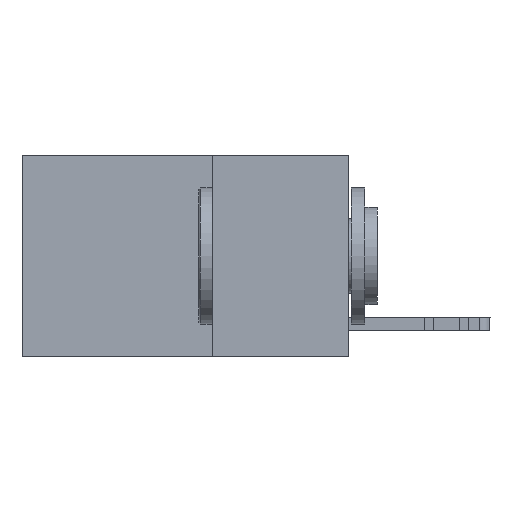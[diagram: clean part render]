
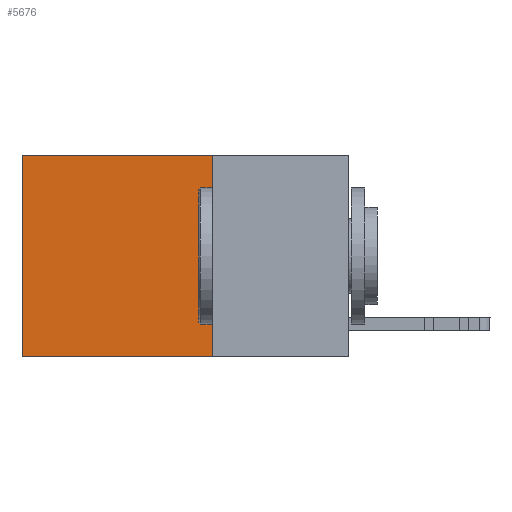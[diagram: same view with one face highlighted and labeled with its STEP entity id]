
A CAD part, left-side view. The second image highlights one B-rep face of the part: STEP entity #5676.
In plain terms, the highlighted planar face has unit normal (-1, 0, 0).
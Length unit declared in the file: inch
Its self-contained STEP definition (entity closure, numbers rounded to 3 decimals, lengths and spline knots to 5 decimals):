
#867 = LINE ( 'NONE', #29846, #5619 ) ;
#2186 = ORIENTED_EDGE ( 'NONE', *, *, #22928, .F. ) ;
#3368 = VERTEX_POINT ( 'NONE', #9059 ) ;
#3508 = ORIENTED_EDGE ( 'NONE', *, *, #18051, .T. ) ;
#5619 = VECTOR ( 'NONE', #25331, 39.37008 ) ;
#5676 = ADVANCED_FACE ( 'NONE', ( #25591 ), #23570, .F. ) ;
#8164 = CARTESIAN_POINT ( 'NONE',  ( 0.2625, 0.6, 0. ) ) ;
#8330 = CARTESIAN_POINT ( 'NONE',  ( 0.2625, 0.6, -0.37 ) ) ;
#8586 = CARTESIAN_POINT ( 'NONE',  ( 0.2625, 0.25, 0. ) ) ;
#9059 = CARTESIAN_POINT ( 'NONE',  ( 0.2625, 0.25, -0.37 ) ) ;
#9687 = CARTESIAN_POINT ( 'NONE',  ( 0.2625, 0.25, 0. ) ) ;
#10790 = CARTESIAN_POINT ( 'NONE',  ( 0.2625, 0.6, 0. ) ) ;
#10986 = VECTOR ( 'NONE', #24557, 39.37008 ) ;
#12030 = DIRECTION ( 'NONE',  ( 0., 0., -1. ) ) ;
#12403 = EDGE_CURVE ( 'NONE', #23217, #15583, #29431, .T. ) ;
#13116 = CARTESIAN_POINT ( 'NONE',  ( 0.2625, 0.25, 0. ) ) ;
#15583 = VERTEX_POINT ( 'NONE', #8330 ) ;
#17139 = VERTEX_POINT ( 'NONE', #8586 ) ;
#17787 = EDGE_CURVE ( 'NONE', #17139, #3368, #23868, .T. ) ;
#18051 = EDGE_CURVE ( 'NONE', #17139, #23217, #24220, .T. ) ;
#19499 = AXIS2_PLACEMENT_3D ( 'NONE', #9687, #25921, #12030 ) ;
#22928 = EDGE_CURVE ( 'NONE', #3368, #15583, #867, .T. ) ;
#23217 = VERTEX_POINT ( 'NONE', #8164 ) ;
#23348 = CARTESIAN_POINT ( 'NONE',  ( 0.2625, 0.25, 0. ) ) ;
#23570 = PLANE ( 'NONE',  #19499 ) ;
#23868 = LINE ( 'NONE', #13116, #29283 ) ;
#24023 = EDGE_LOOP ( 'NONE', ( #29647, #2186, #27839, #3508 ) ) ;
#24220 = LINE ( 'NONE', #23348, #28920 ) ;
#24557 = DIRECTION ( 'NONE',  ( 0., 0., -1. ) ) ;
#25331 = DIRECTION ( 'NONE',  ( 0., 1., 0. ) ) ;
#25591 = FACE_OUTER_BOUND ( 'NONE', #24023, .T. ) ;
#25694 = DIRECTION ( 'NONE',  ( 0., 1., 0. ) ) ;
#25921 = DIRECTION ( 'NONE',  ( 1., 0., 0. ) ) ;
#27113 = DIRECTION ( 'NONE',  ( 0., 0., -1. ) ) ;
#27839 = ORIENTED_EDGE ( 'NONE', *, *, #17787, .F. ) ;
#28920 = VECTOR ( 'NONE', #25694, 39.37008 ) ;
#29283 = VECTOR ( 'NONE', #27113, 39.37008 ) ;
#29431 = LINE ( 'NONE', #10790, #10986 ) ;
#29647 = ORIENTED_EDGE ( 'NONE', *, *, #12403, .T. ) ;
#29846 = CARTESIAN_POINT ( 'NONE',  ( 0.2625, 0.25, -0.37 ) ) ;
